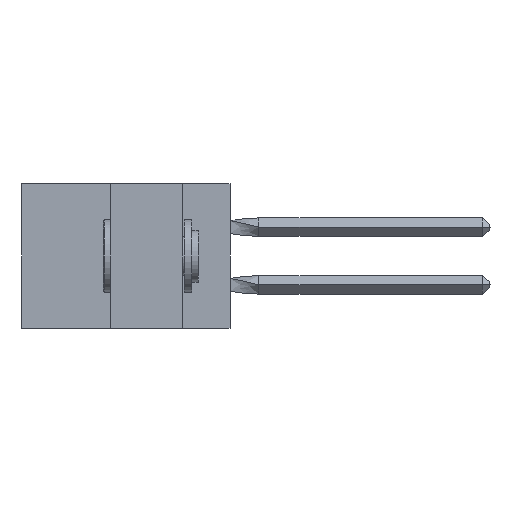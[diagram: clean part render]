
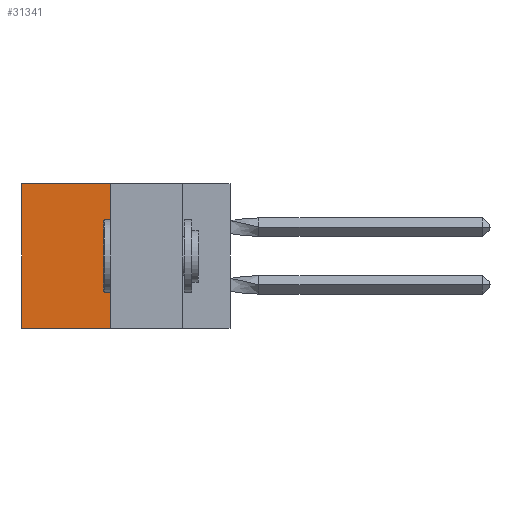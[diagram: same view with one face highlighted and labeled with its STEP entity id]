
A CAD part, left-side view. The second image highlights one B-rep face of the part: STEP entity #31341.
In plain terms, the highlighted planar face has unit normal (-1, 0, 0).
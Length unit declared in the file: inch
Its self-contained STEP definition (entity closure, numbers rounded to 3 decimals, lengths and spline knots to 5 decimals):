
#23 = CARTESIAN_POINT ( 'NONE',  ( 0.305, 0.413, 0. ) ) ;
#1151 = DIRECTION ( 'NONE',  ( 1., 0., 0. ) ) ;
#2220 = VECTOR ( 'NONE', #8531, 39.37008 ) ;
#3440 = CARTESIAN_POINT ( 'NONE',  ( 0.305, 0.72, -0.5 ) ) ;
#3766 = PLANE ( 'NONE',  #16651 ) ;
#3941 = LINE ( 'NONE', #24686, #2220 ) ;
#4394 = ORIENTED_EDGE ( 'NONE', *, *, #13923, .F. ) ;
#4733 = FACE_OUTER_BOUND ( 'NONE', #8289, .T. ) ;
#6264 = DIRECTION ( 'NONE',  ( 0., 0., -1. ) ) ;
#6670 = ORIENTED_EDGE ( 'NONE', *, *, #30057, .T. ) ;
#6687 = VECTOR ( 'NONE', #10975, 39.37008 ) ;
#6758 = ORIENTED_EDGE ( 'NONE', *, *, #32644, .T. ) ;
#6774 = VERTEX_POINT ( 'NONE', #13752 ) ;
#8289 = EDGE_LOOP ( 'NONE', ( #6758, #34721, #4394, #6670 ) ) ;
#8531 = DIRECTION ( 'NONE',  ( 0., 1., 0. ) ) ;
#9430 = VECTOR ( 'NONE', #16251, 39.37008 ) ;
#9964 = EDGE_CURVE ( 'NONE', #6774, #31374, #3941, .T. ) ;
#10727 = CARTESIAN_POINT ( 'NONE',  ( 0.305, 0.413, 0. ) ) ;
#10796 = CARTESIAN_POINT ( 'NONE',  ( 0.305, 0.72, -0.5 ) ) ;
#10975 = DIRECTION ( 'NONE',  ( 0., 1., 0. ) ) ;
#13752 = CARTESIAN_POINT ( 'NONE',  ( 0.305, 0.413, -0.5 ) ) ;
#13923 = EDGE_CURVE ( 'NONE', #32806, #6774, #15542, .T. ) ;
#15542 = LINE ( 'NONE', #24542, #32124 ) ;
#16251 = DIRECTION ( 'NONE',  ( 0., 0., -1. ) ) ;
#16651 = AXIS2_PLACEMENT_3D ( 'NONE', #33715, #1151, #6264 ) ;
#17083 = LINE ( 'NONE', #10796, #9430 ) ;
#17348 = LINE ( 'NONE', #10727, #6687 ) ;
#18890 = VERTEX_POINT ( 'NONE', #27361 ) ;
#24542 = CARTESIAN_POINT ( 'NONE',  ( 0.305, 0.413, -0.5 ) ) ;
#24686 = CARTESIAN_POINT ( 'NONE',  ( 0.305, 0.413, -0.5 ) ) ;
#27361 = CARTESIAN_POINT ( 'NONE',  ( 0.305, 0.72, 0. ) ) ;
#30057 = EDGE_CURVE ( 'NONE', #32806, #18890, #17348, .T. ) ;
#31341 = ADVANCED_FACE ( 'NONE', ( #4733 ), #3766, .F. ) ;
#31374 = VERTEX_POINT ( 'NONE', #3440 ) ;
#32124 = VECTOR ( 'NONE', #33207, 39.37008 ) ;
#32644 = EDGE_CURVE ( 'NONE', #18890, #31374, #17083, .T. ) ;
#32806 = VERTEX_POINT ( 'NONE', #23 ) ;
#33207 = DIRECTION ( 'NONE',  ( 0., 0., -1. ) ) ;
#33715 = CARTESIAN_POINT ( 'NONE',  ( 0.305, 0.413, -0.5 ) ) ;
#34721 = ORIENTED_EDGE ( 'NONE', *, *, #9964, .F. ) ;
